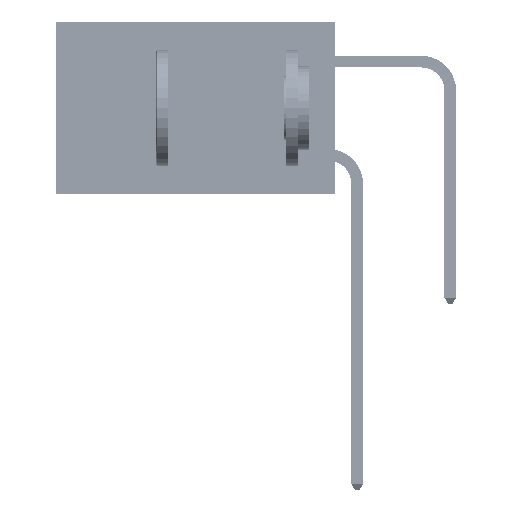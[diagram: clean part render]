
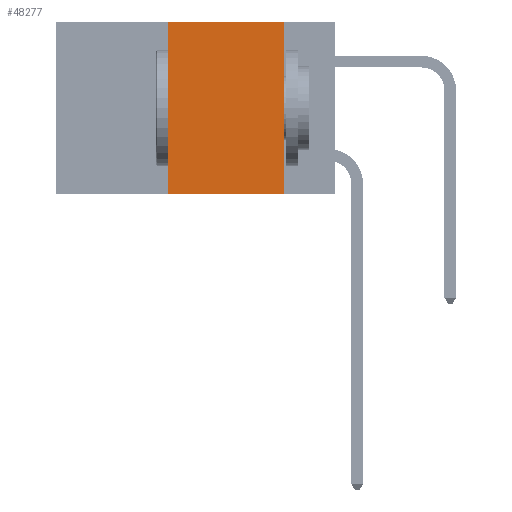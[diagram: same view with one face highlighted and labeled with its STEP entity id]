
A CAD part, left-side view. The second image highlights one B-rep face of the part: STEP entity #48277.
In plain terms, the highlighted planar face has unit normal (-1, 0, 0).
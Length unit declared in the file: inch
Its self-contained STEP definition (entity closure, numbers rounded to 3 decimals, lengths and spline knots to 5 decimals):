
#187 = FACE_OUTER_BOUND ( 'NONE', #16781, .T. ) ;
#437 = EDGE_CURVE ( 'NONE', #36136, #51737, #950, .T. ) ;
#495 = DIRECTION ( 'NONE',  ( 0., 0., 1. ) ) ;
#950 = LINE ( 'NONE', #9119, #10150 ) ;
#1631 = EDGE_CURVE ( 'NONE', #36136, #36781, #25769, .T. ) ;
#3445 = CARTESIAN_POINT ( 'NONE',  ( 0., 0.6, 0. ) ) ;
#4641 = EDGE_CURVE ( 'NONE', #51737, #38341, #10939, .T. ) ;
#9119 = CARTESIAN_POINT ( 'NONE',  ( 0., 0.36, 0. ) ) ;
#9764 = CARTESIAN_POINT ( 'NONE',  ( 0., 0.11, 0. ) ) ;
#10150 = VECTOR ( 'NONE', #495, 39.37008 ) ;
#10939 = LINE ( 'NONE', #40353, #29356 ) ;
#13158 = AXIS2_PLACEMENT_3D ( 'NONE', #3445, #20695, #28771 ) ;
#16748 = ORIENTED_EDGE ( 'NONE', *, *, #4641, .F. ) ;
#16781 = EDGE_LOOP ( 'NONE', ( #35081, #16748, #32295, #20880 ) ) ;
#18972 = CARTESIAN_POINT ( 'NONE',  ( 0., 0.36, -0.37 ) ) ;
#19174 = VECTOR ( 'NONE', #24621, 39.37008 ) ;
#20027 = CARTESIAN_POINT ( 'NONE',  ( 0., 0.6, -0.37 ) ) ;
#20695 = DIRECTION ( 'NONE',  ( 1., 0., 0. ) ) ;
#20880 = ORIENTED_EDGE ( 'NONE', *, *, #1631, .T. ) ;
#23862 = EDGE_CURVE ( 'NONE', #38341, #36781, #48868, .T. ) ;
#24621 = DIRECTION ( 'NONE',  ( 0., -1., 0. ) ) ;
#25769 = LINE ( 'NONE', #20027, #19174 ) ;
#26142 = DIRECTION ( 'NONE',  ( 0., 0., -1. ) ) ;
#27815 = CARTESIAN_POINT ( 'NONE',  ( 0., 0.11, 0. ) ) ;
#28586 = PLANE ( 'NONE',  #13158 ) ;
#28771 = DIRECTION ( 'NONE',  ( 0., 0., -1. ) ) ;
#29175 = CARTESIAN_POINT ( 'NONE',  ( 0., 0.36, 0. ) ) ;
#29356 = VECTOR ( 'NONE', #33192, 39.37008 ) ;
#31878 = VECTOR ( 'NONE', #26142, 39.37008 ) ;
#32295 = ORIENTED_EDGE ( 'NONE', *, *, #437, .F. ) ;
#33192 = DIRECTION ( 'NONE',  ( 0., -1., 0. ) ) ;
#35081 = ORIENTED_EDGE ( 'NONE', *, *, #23862, .F. ) ;
#35413 = CARTESIAN_POINT ( 'NONE',  ( 0., 0.11, -0.37 ) ) ;
#36136 = VERTEX_POINT ( 'NONE', #18972 ) ;
#36781 = VERTEX_POINT ( 'NONE', #35413 ) ;
#38341 = VERTEX_POINT ( 'NONE', #27815 ) ;
#40353 = CARTESIAN_POINT ( 'NONE',  ( 0., 0.6, 0. ) ) ;
#48277 = ADVANCED_FACE ( 'NONE', ( #187 ), #28586, .F. ) ;
#48868 = LINE ( 'NONE', #9764, #31878 ) ;
#51737 = VERTEX_POINT ( 'NONE', #29175 ) ;
